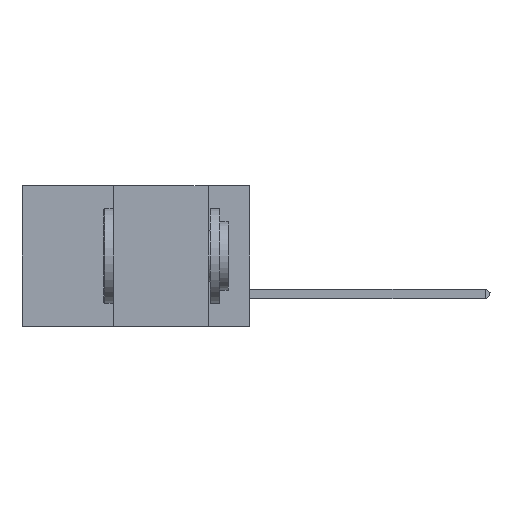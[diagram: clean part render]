
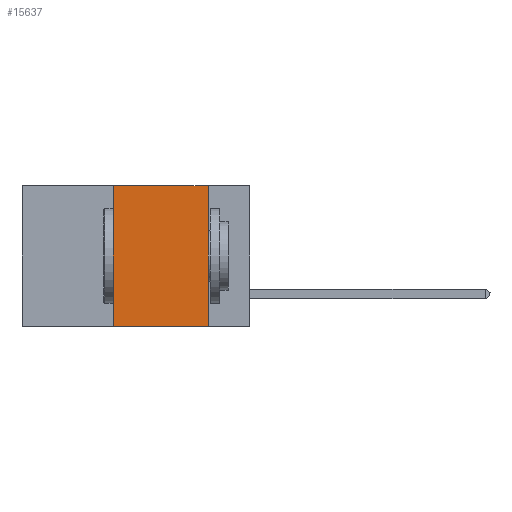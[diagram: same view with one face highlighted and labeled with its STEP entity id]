
A CAD part, left-side view. The second image highlights one B-rep face of the part: STEP entity #15637.
In plain terms, the highlighted planar face has unit normal (-1, 0, 0).
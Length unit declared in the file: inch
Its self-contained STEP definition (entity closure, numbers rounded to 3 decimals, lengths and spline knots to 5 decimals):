
#1716 = DIRECTION ( 'NONE',  ( 0., 0., -1. ) ) ;
#1925 = VERTEX_POINT ( 'NONE', #29357 ) ;
#2397 = ORIENTED_EDGE ( 'NONE', *, *, #19852, .F. ) ;
#2705 = CARTESIAN_POINT ( 'NONE',  ( 0., 0.36, -0.37 ) ) ;
#2867 = LINE ( 'NONE', #30676, #15065 ) ;
#4905 = ORIENTED_EDGE ( 'NONE', *, *, #23295, .F. ) ;
#5061 = VECTOR ( 'NONE', #7601, 39.37008 ) ;
#5627 = VECTOR ( 'NONE', #42026, 39.37008 ) ;
#7601 = DIRECTION ( 'NONE',  ( 0., -1., 0. ) ) ;
#8011 = PLANE ( 'NONE',  #14769 ) ;
#9874 = ORIENTED_EDGE ( 'NONE', *, *, #26682, .T. ) ;
#10787 = EDGE_CURVE ( 'NONE', #29810, #1925, #33211, .T. ) ;
#11434 = ORIENTED_EDGE ( 'NONE', *, *, #10787, .F. ) ;
#13828 = CARTESIAN_POINT ( 'NONE',  ( 0., 0.6, -0.37 ) ) ;
#14215 = VERTEX_POINT ( 'NONE', #17503 ) ;
#14729 = CARTESIAN_POINT ( 'NONE',  ( 0., 0.11, -0.37 ) ) ;
#14769 = AXIS2_PLACEMENT_3D ( 'NONE', #21368, #28199, #1716 ) ;
#15065 = VECTOR ( 'NONE', #19499, 39.37008 ) ;
#15637 = ADVANCED_FACE ( 'NONE', ( #24698 ), #8011, .F. ) ;
#17503 = CARTESIAN_POINT ( 'NONE',  ( 0., 0.11, 0. ) ) ;
#19132 = CARTESIAN_POINT ( 'NONE',  ( 0., 0.6, 0. ) ) ;
#19499 = DIRECTION ( 'NONE',  ( 0., 0., -1. ) ) ;
#19852 = EDGE_CURVE ( 'NONE', #14215, #39585, #2867, .T. ) ;
#21368 = CARTESIAN_POINT ( 'NONE',  ( 0., 0.6, 0. ) ) ;
#23295 = EDGE_CURVE ( 'NONE', #1925, #14215, #30002, .T. ) ;
#24698 = FACE_OUTER_BOUND ( 'NONE', #39892, .T. ) ;
#26682 = EDGE_CURVE ( 'NONE', #29810, #39585, #37186, .T. ) ;
#28199 = DIRECTION ( 'NONE',  ( 1., 0., 0. ) ) ;
#29357 = CARTESIAN_POINT ( 'NONE',  ( 0., 0.36, 0. ) ) ;
#29810 = VERTEX_POINT ( 'NONE', #2705 ) ;
#30002 = LINE ( 'NONE', #19132, #5627 ) ;
#30676 = CARTESIAN_POINT ( 'NONE',  ( 0., 0.11, 0. ) ) ;
#32387 = CARTESIAN_POINT ( 'NONE',  ( 0., 0.36, 0. ) ) ;
#32747 = VECTOR ( 'NONE', #39497, 39.37008 ) ;
#33211 = LINE ( 'NONE', #32387, #32747 ) ;
#37186 = LINE ( 'NONE', #13828, #5061 ) ;
#39497 = DIRECTION ( 'NONE',  ( 0., 0., 1. ) ) ;
#39585 = VERTEX_POINT ( 'NONE', #14729 ) ;
#39892 = EDGE_LOOP ( 'NONE', ( #2397, #4905, #11434, #9874 ) ) ;
#42026 = DIRECTION ( 'NONE',  ( 0., -1., 0. ) ) ;
